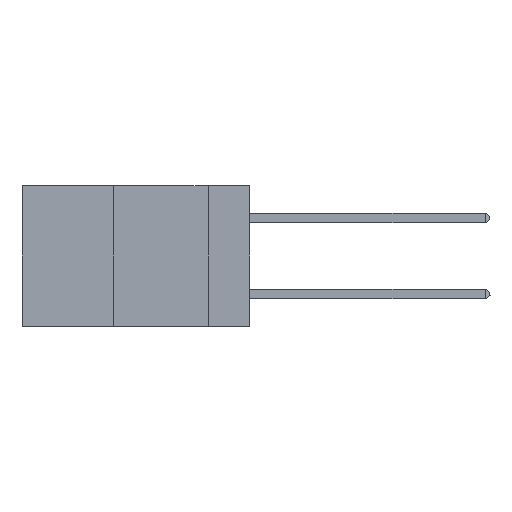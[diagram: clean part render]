
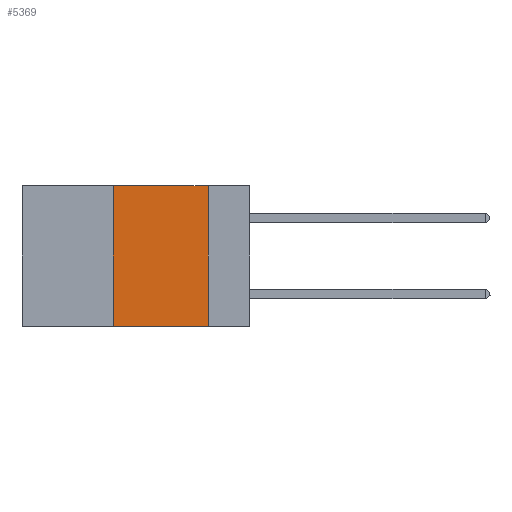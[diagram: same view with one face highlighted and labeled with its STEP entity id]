
A CAD part, left-side view. The second image highlights one B-rep face of the part: STEP entity #5369.
In plain terms, the highlighted planar face has unit normal (-1, 0, 0).
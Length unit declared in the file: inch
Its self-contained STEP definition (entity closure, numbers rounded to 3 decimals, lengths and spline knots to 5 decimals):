
#3574 = AXIS2_PLACEMENT_3D ( 'NONE', #36586, #23830, #14040 ) ;
#4504 = ORIENTED_EDGE ( 'NONE', *, *, #32342, .F. ) ;
#5012 = ORIENTED_EDGE ( 'NONE', *, *, #32523, .F. ) ;
#5296 = VERTEX_POINT ( 'NONE', #35750 ) ;
#5369 = ADVANCED_FACE ( 'NONE', ( #17799 ), #33361, .F. ) ;
#5893 = CARTESIAN_POINT ( 'NONE',  ( 0., 0.36, 0. ) ) ;
#8129 = CARTESIAN_POINT ( 'NONE',  ( 0., 0.36, 0. ) ) ;
#8232 = DIRECTION ( 'NONE',  ( 0., -1., 0. ) ) ;
#10124 = ORIENTED_EDGE ( 'NONE', *, *, #10614, .F. ) ;
#10614 = EDGE_CURVE ( 'NONE', #22736, #38711, #37942, .T. ) ;
#10728 = LINE ( 'NONE', #36851, #22716 ) ;
#13564 = CARTESIAN_POINT ( 'NONE',  ( 0., 0.6, -0.37 ) ) ;
#14040 = DIRECTION ( 'NONE',  ( 0., 0., -1. ) ) ;
#16237 = VECTOR ( 'NONE', #18238, 39.37008 ) ;
#17799 = FACE_OUTER_BOUND ( 'NONE', #21146, .T. ) ;
#18238 = DIRECTION ( 'NONE',  ( 0., 0., 1. ) ) ;
#18912 = VECTOR ( 'NONE', #8232, 39.37008 ) ;
#19982 = DIRECTION ( 'NONE',  ( 0., -1., 0. ) ) ;
#21146 = EDGE_LOOP ( 'NONE', ( #4504, #10124, #5012, #33492 ) ) ;
#22716 = VECTOR ( 'NONE', #36712, 39.37008 ) ;
#22736 = VERTEX_POINT ( 'NONE', #5893 ) ;
#23830 = DIRECTION ( 'NONE',  ( 1., 0., 0. ) ) ;
#26555 = LINE ( 'NONE', #13564, #40592 ) ;
#26739 = LINE ( 'NONE', #8129, #16237 ) ;
#28240 = EDGE_CURVE ( 'NONE', #37914, #5296, #26555, .T. ) ;
#32342 = EDGE_CURVE ( 'NONE', #38711, #5296, #10728, .T. ) ;
#32523 = EDGE_CURVE ( 'NONE', #37914, #22736, #26739, .T. ) ;
#33287 = CARTESIAN_POINT ( 'NONE',  ( 0., 0.11, 0. ) ) ;
#33361 = PLANE ( 'NONE',  #3574 ) ;
#33452 = CARTESIAN_POINT ( 'NONE',  ( 0., 0.6, 0. ) ) ;
#33492 = ORIENTED_EDGE ( 'NONE', *, *, #28240, .T. ) ;
#35750 = CARTESIAN_POINT ( 'NONE',  ( 0., 0.11, -0.37 ) ) ;
#36018 = CARTESIAN_POINT ( 'NONE',  ( 0., 0.36, -0.37 ) ) ;
#36586 = CARTESIAN_POINT ( 'NONE',  ( 0., 0.6, 0. ) ) ;
#36712 = DIRECTION ( 'NONE',  ( 0., 0., -1. ) ) ;
#36851 = CARTESIAN_POINT ( 'NONE',  ( 0., 0.11, 0. ) ) ;
#37914 = VERTEX_POINT ( 'NONE', #36018 ) ;
#37942 = LINE ( 'NONE', #33452, #18912 ) ;
#38711 = VERTEX_POINT ( 'NONE', #33287 ) ;
#40592 = VECTOR ( 'NONE', #19982, 39.37008 ) ;
